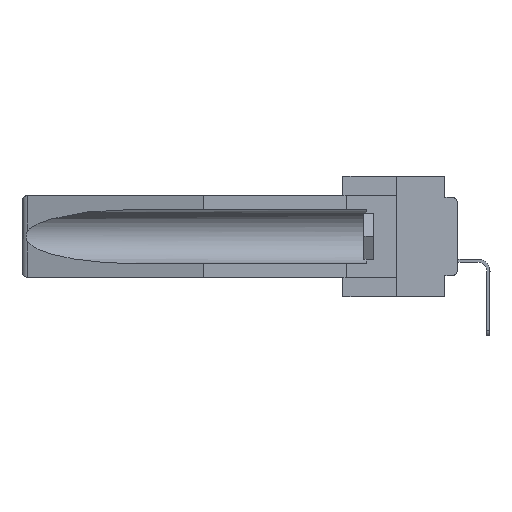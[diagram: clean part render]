
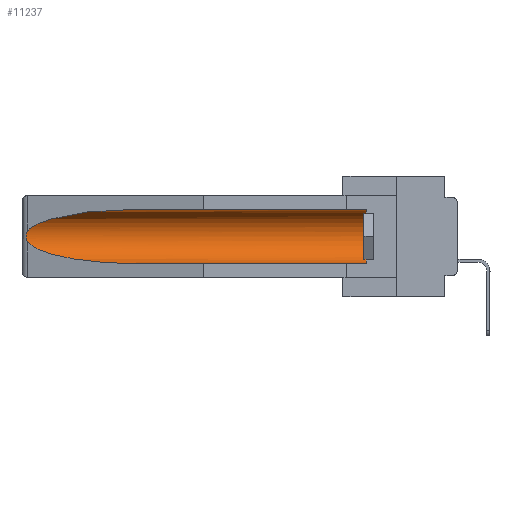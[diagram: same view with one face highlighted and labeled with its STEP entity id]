
A CAD part, left-side view. The second image highlights one B-rep face of the part: STEP entity #11237.
In plain terms, the highlighted cylindrical face has radius 2.857 mm (diameter 5.715 mm), a partial arc.
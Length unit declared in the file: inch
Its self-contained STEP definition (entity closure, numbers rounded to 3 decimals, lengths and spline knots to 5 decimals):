
#708 = CARTESIAN_POINT ( 'NONE',  ( 0.155, 1.07973, -0.284 ) ) ;
#1127 = ORIENTED_EDGE ( 'NONE', *, *, #1708, .T. ) ;
#1708 = EDGE_CURVE ( 'NONE', #35993, #10130, #18513, .T. ) ;
#2188 = CARTESIAN_POINT ( 'NONE',  ( 0.26597, 1.52961, -0.15275 ) ) ;
#2313 = CARTESIAN_POINT ( 'NONE',  ( 0.26654, 1.53092, -0.15636 ) ) ;
#4515 = FACE_OUTER_BOUND ( 'NONE', #13850, .T. ) ;
#4631 = CARTESIAN_POINT ( 'NONE',  ( 0.155, 1.07973, -0.284 ) ) ;
#4904 = DIRECTION ( 'NONE',  ( 0., -1., 0. ) ) ;
#5023 = CARTESIAN_POINT ( 'NONE',  ( 0.2675, 1.53308, -0.17534 ) ) ;
#5139 = CARTESIAN_POINT ( 'NONE',  ( 0.26597, 1.5296, -0.19026 ) ) ;
#6584 = EDGE_CURVE ( 'NONE', #16874, #35993, #23021, .T. ) ;
#7159 = CYLINDRICAL_SURFACE ( 'NONE', #16809, 0.1125 ) ;
#8161 = CARTESIAN_POINT ( 'NONE',  ( 0.155, 0.126, -0.284 ) ) ;
#8354 = LINE ( 'NONE', #28772, #23746 ) ;
#8416 = EDGE_CURVE ( 'NONE', #15813, #20727, #18466, .T. ) ;
#9369 = CARTESIAN_POINT ( 'NONE',  ( 0.155, -0.30754, -0.059 ) ) ;
#10028 = ORIENTED_EDGE ( 'NONE', *, *, #18046, .T. ) ;
#10130 = VERTEX_POINT ( 'NONE', #19205 ) ;
#10727 = ORIENTED_EDGE ( 'NONE', *, *, #6584, .T. ) ;
#10822 = DIRECTION ( 'NONE',  ( 0., 1., 0. ) ) ;
#11237 = ADVANCED_FACE ( 'NONE', ( #4515 ), #7159, .F. ) ;
#12092 = CARTESIAN_POINT ( 'NONE',  ( 0.21114, 1.30732, -0.284 ) ) ;
#13493 = CARTESIAN_POINT ( 'NONE',  ( 0.2673, 1.53269, -0.17917 ) ) ;
#13830 = CARTESIAN_POINT ( 'NONE',  ( 0.26537, 1.52718, -0.14972 ) ) ;
#13850 = EDGE_LOOP ( 'NONE', ( #1127, #10028, #34387, #22517, #34848, #10727 ) ) ;
#15261 = DIRECTION ( 'NONE',  ( 0., 0., 1. ) ) ;
#15534 = VECTOR ( 'NONE', #17230, 39.37008 ) ;
#15542 = VERTEX_POINT ( 'NONE', #8161 ) ;
#15621 = CARTESIAN_POINT ( 'NONE',  ( 0.155, 1.07973, -0.059 ) ) ;
#15813 = VERTEX_POINT ( 'NONE', #34518 ) ;
#16284 = CARTESIAN_POINT ( 'NONE',  ( 0.155, 1.07973, -0.059 ) ) ;
#16809 = AXIS2_PLACEMENT_3D ( 'NONE', #30231, #10822, #15261 ) ;
#16874 = VERTEX_POINT ( 'NONE', #33964 ) ;
#17230 = DIRECTION ( 'NONE',  ( 0., 1., 0. ) ) ;
#18046 = EDGE_CURVE ( 'NONE', #10130, #15813, #21178, .T. ) ;
#18466 =( BOUNDED_CURVE ( )  B_SPLINE_CURVE ( 3, ( #28804, #23517, #12092, #708 ),
 .UNSPECIFIED., .F., .F. ) 
 B_SPLINE_CURVE_WITH_KNOTS ( ( 4, 4 ),
 ( 0.1948, 1.5708 ),
 .UNSPECIFIED. ) 
 CURVE ( )  GEOMETRIC_REPRESENTATION_ITEM ( )  RATIONAL_B_SPLINE_CURVE ( ( 1., 0.848, 0.848, 1. ) ) 
 REPRESENTATION_ITEM ( '' )  );
#18513 =( BOUNDED_CURVE ( )  B_SPLINE_CURVE ( 3, ( #16284, #21925, #24625, #13830 ),
 .UNSPECIFIED., .F., .F. ) 
 B_SPLINE_CURVE_WITH_KNOTS ( ( 4, 4 ),
 ( 4.71239, 6.08839 ),
 .UNSPECIFIED. ) 
 CURVE ( )  GEOMETRIC_REPRESENTATION_ITEM ( )  RATIONAL_B_SPLINE_CURVE ( ( 1., 0.848, 0.848, 1. ) ) 
 REPRESENTATION_ITEM ( '' )  );
#19205 = CARTESIAN_POINT ( 'NONE',  ( 0.26537, 1.52718, -0.14972 ) ) ;
#20400 = CIRCLE ( 'NONE', #27211, 0.1125 ) ;
#20727 = VERTEX_POINT ( 'NONE', #4631 ) ;
#21178 = B_SPLINE_CURVE_WITH_KNOTS ( 'NONE', 3,
 ( #32873, #2188, #2313, #35943, #30306, #5023, #13493, #24865, #5139, #33118 ),
 .UNSPECIFIED., .F., .F.,
 ( 4, 2, 2, 2, 4 ),
 ( 0., 0.00029, 0.00058, 0.00087, 0.00117 ),
 .UNSPECIFIED. ) ;
#21925 = CARTESIAN_POINT ( 'NONE',  ( 0.21114, 1.30732, -0.059 ) ) ;
#22517 = ORIENTED_EDGE ( 'NONE', *, *, #25330, .F. ) ;
#23021 = LINE ( 'NONE', #9369, #15534 ) ;
#23517 = CARTESIAN_POINT ( 'NONE',  ( 0.25451, 1.48313, -0.24835 ) ) ;
#23746 = VECTOR ( 'NONE', #29011, 39.37008 ) ;
#24625 = CARTESIAN_POINT ( 'NONE',  ( 0.25451, 1.48313, -0.09465 ) ) ;
#24865 = CARTESIAN_POINT ( 'NONE',  ( 0.26655, 1.53094, -0.18657 ) ) ;
#25330 = EDGE_CURVE ( 'NONE', #15542, #20727, #8354, .T. ) ;
#27211 = AXIS2_PLACEMENT_3D ( 'NONE', #32880, #4904, #32395 ) ;
#28772 = CARTESIAN_POINT ( 'NONE',  ( 0.155, -0.30754, -0.284 ) ) ;
#28804 = CARTESIAN_POINT ( 'NONE',  ( 0.26537, 1.52718, -0.19328 ) ) ;
#29011 = DIRECTION ( 'NONE',  ( 0., 1., 0. ) ) ;
#29935 = EDGE_CURVE ( 'NONE', #15542, #16874, #20400, .T. ) ;
#30231 = CARTESIAN_POINT ( 'NONE',  ( 0.155, -0.30754, -0.1715 ) ) ;
#30306 = CARTESIAN_POINT ( 'NONE',  ( 0.2675, 1.53308, -0.16763 ) ) ;
#32395 = DIRECTION ( 'NONE',  ( 0., 0., 1. ) ) ;
#32873 = CARTESIAN_POINT ( 'NONE',  ( 0.26537, 1.52718, -0.14972 ) ) ;
#32880 = CARTESIAN_POINT ( 'NONE',  ( 0.155, 0.126, -0.1715 ) ) ;
#33118 = CARTESIAN_POINT ( 'NONE',  ( 0.26537, 1.52718, -0.19328 ) ) ;
#33964 = CARTESIAN_POINT ( 'NONE',  ( 0.155, 0.126, -0.059 ) ) ;
#34387 = ORIENTED_EDGE ( 'NONE', *, *, #8416, .T. ) ;
#34518 = CARTESIAN_POINT ( 'NONE',  ( 0.26537, 1.52718, -0.19328 ) ) ;
#34848 = ORIENTED_EDGE ( 'NONE', *, *, #29935, .T. ) ;
#35943 = CARTESIAN_POINT ( 'NONE',  ( 0.2673, 1.5327, -0.16383 ) ) ;
#35993 = VERTEX_POINT ( 'NONE', #15621 ) ;
